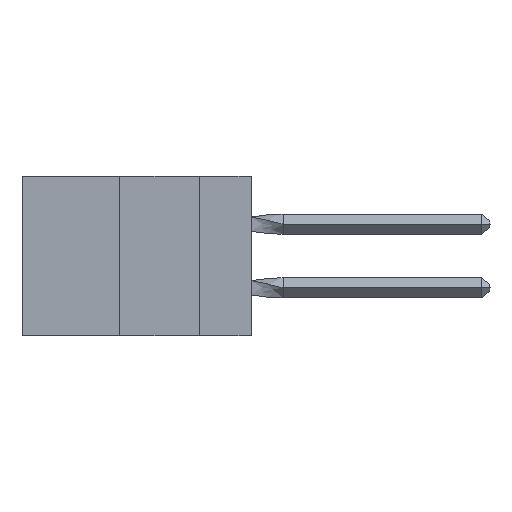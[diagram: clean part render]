
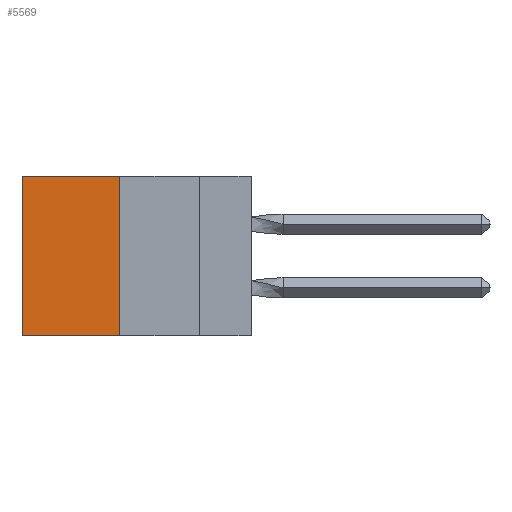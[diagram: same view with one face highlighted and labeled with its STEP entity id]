
A CAD part, left-side view. The second image highlights one B-rep face of the part: STEP entity #5569.
In plain terms, the highlighted planar face has unit normal (-1, 0, 0).
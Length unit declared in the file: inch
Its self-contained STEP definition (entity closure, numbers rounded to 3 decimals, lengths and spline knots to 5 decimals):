
#523 = DIRECTION ( 'NONE',  ( 0., 0., -1. ) ) ;
#1006 = ORIENTED_EDGE ( 'NONE', *, *, #3496, .T. ) ;
#1191 = EDGE_CURVE ( 'NONE', #6445, #16763, #23989, .T. ) ;
#1270 = FACE_OUTER_BOUND ( 'NONE', #26590, .T. ) ;
#1418 = DIRECTION ( 'NONE',  ( 0., 1., 0. ) ) ;
#2023 = CARTESIAN_POINT ( 'NONE',  ( 0.305, 0.413, -0.5 ) ) ;
#2498 = EDGE_CURVE ( 'NONE', #23400, #9893, #23261, .T. ) ;
#2843 = ORIENTED_EDGE ( 'NONE', *, *, #2498, .F. ) ;
#3496 = EDGE_CURVE ( 'NONE', #23400, #6445, #17259, .T. ) ;
#5221 = DIRECTION ( 'NONE',  ( 0., 0., -1. ) ) ;
#5569 = ADVANCED_FACE ( 'NONE', ( #1270 ), #24224, .F. ) ;
#6137 = DIRECTION ( 'NONE',  ( 0., 1., 0. ) ) ;
#6445 = VERTEX_POINT ( 'NONE', #29181 ) ;
#7776 = CARTESIAN_POINT ( 'NONE',  ( 0.305, 0.413, -0.5 ) ) ;
#8981 = CARTESIAN_POINT ( 'NONE',  ( 0.305, 0.72, -0.5 ) ) ;
#9372 = EDGE_CURVE ( 'NONE', #9893, #16763, #15994, .T. ) ;
#9893 = VERTEX_POINT ( 'NONE', #2023 ) ;
#10168 = DIRECTION ( 'NONE',  ( 1., 0., 0. ) ) ;
#10361 = ORIENTED_EDGE ( 'NONE', *, *, #1191, .T. ) ;
#10918 = CARTESIAN_POINT ( 'NONE',  ( 0.305, 0.413, 0. ) ) ;
#10985 = AXIS2_PLACEMENT_3D ( 'NONE', #7776, #10168, #5221 ) ;
#13696 = DIRECTION ( 'NONE',  ( 0., 0., -1. ) ) ;
#13772 = VECTOR ( 'NONE', #1418, 39.37008 ) ;
#15994 = LINE ( 'NONE', #17877, #13772 ) ;
#16763 = VERTEX_POINT ( 'NONE', #8981 ) ;
#17259 = LINE ( 'NONE', #23095, #29821 ) ;
#17401 = ORIENTED_EDGE ( 'NONE', *, *, #9372, .F. ) ;
#17877 = CARTESIAN_POINT ( 'NONE',  ( 0.305, 0.413, -0.5 ) ) ;
#23095 = CARTESIAN_POINT ( 'NONE',  ( 0.305, 0.413, 0. ) ) ;
#23261 = LINE ( 'NONE', #24215, #24384 ) ;
#23400 = VERTEX_POINT ( 'NONE', #10918 ) ;
#23592 = VECTOR ( 'NONE', #523, 39.37008 ) ;
#23989 = LINE ( 'NONE', #25793, #23592 ) ;
#24215 = CARTESIAN_POINT ( 'NONE',  ( 0.305, 0.413, -0.5 ) ) ;
#24224 = PLANE ( 'NONE',  #10985 ) ;
#24384 = VECTOR ( 'NONE', #13696, 39.37008 ) ;
#25793 = CARTESIAN_POINT ( 'NONE',  ( 0.305, 0.72, -0.5 ) ) ;
#26590 = EDGE_LOOP ( 'NONE', ( #10361, #17401, #2843, #1006 ) ) ;
#29181 = CARTESIAN_POINT ( 'NONE',  ( 0.305, 0.72, 0. ) ) ;
#29821 = VECTOR ( 'NONE', #6137, 39.37008 ) ;
